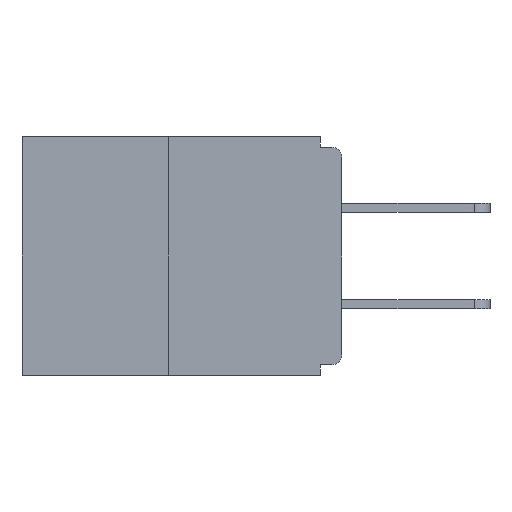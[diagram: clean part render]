
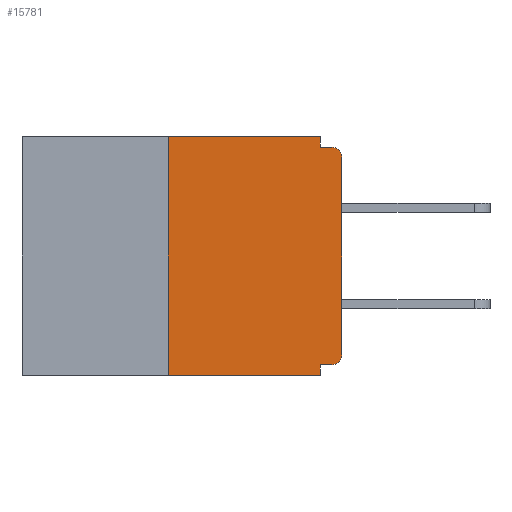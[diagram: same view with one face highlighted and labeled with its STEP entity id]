
A CAD part, left-side view. The second image highlights one B-rep face of the part: STEP entity #15781.
In plain terms, the highlighted planar face has unit normal (-1, 0, 0).
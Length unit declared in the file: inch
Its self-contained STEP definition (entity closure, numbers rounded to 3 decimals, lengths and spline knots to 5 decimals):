
#183 = CARTESIAN_POINT ( 'NONE',  ( 0., 0.46, 0. ) ) ;
#413 = ORIENTED_EDGE ( 'NONE', *, *, #6969, .F. ) ;
#437 = DIRECTION ( 'NONE',  ( 0., 0., -1. ) ) ;
#594 = VECTOR ( 'NONE', #13583, 39.37008 ) ;
#1017 = CIRCLE ( 'NONE', #13633, 0.015 ) ;
#1108 = VERTEX_POINT ( 'NONE', #19382 ) ;
#1325 = CARTESIAN_POINT ( 'NONE',  ( 0., 0.46, 0. ) ) ;
#1712 = FACE_OUTER_BOUND ( 'NONE', #11593, .T. ) ;
#1783 = PLANE ( 'NONE',  #17077 ) ;
#1824 = CARTESIAN_POINT ( 'NONE',  ( 0., 0., -0.015 ) ) ;
#2771 = CARTESIAN_POINT ( 'NONE',  ( 0., 0., 0. ) ) ;
#2826 = CARTESIAN_POINT ( 'NONE',  ( 0., 0.015, -0.03 ) ) ;
#3890 = ORIENTED_EDGE ( 'NONE', *, *, #14543, .F. ) ;
#4181 = EDGE_CURVE ( 'NONE', #9785, #1108, #5140, .T. ) ;
#4835 = CARTESIAN_POINT ( 'NONE',  ( 0., 0.031, 0. ) ) ;
#5004 = CARTESIAN_POINT ( 'NONE',  ( 0., 0.031, -0.328 ) ) ;
#5140 = LINE ( 'NONE', #2771, #10177 ) ;
#5144 = LINE ( 'NONE', #1824, #17123 ) ;
#6903 = VECTOR ( 'NONE', #10868, 39.37008 ) ;
#6969 = EDGE_CURVE ( 'NONE', #14451, #9485, #12203, .T. ) ;
#7129 = VERTEX_POINT ( 'NONE', #18935 ) ;
#7306 = VECTOR ( 'NONE', #13281, 39.37008 ) ;
#7949 = DIRECTION ( 'NONE',  ( 0., 0., -1. ) ) ;
#7967 = ORIENTED_EDGE ( 'NONE', *, *, #14686, .F. ) ;
#8321 = VERTEX_POINT ( 'NONE', #12087 ) ;
#8353 = CARTESIAN_POINT ( 'NONE',  ( 0., 0.031, 0. ) ) ;
#8525 = EDGE_CURVE ( 'NONE', #9485, #16801, #18585, .T. ) ;
#8793 = CARTESIAN_POINT ( 'NONE',  ( 0., 0., -0.313 ) ) ;
#9000 = EDGE_CURVE ( 'NONE', #19195, #7129, #12883, .T. ) ;
#9148 = ORIENTED_EDGE ( 'NONE', *, *, #10459, .T. ) ;
#9485 = VERTEX_POINT ( 'NONE', #4835 ) ;
#9785 = VERTEX_POINT ( 'NONE', #8793 ) ;
#10020 = LINE ( 'NONE', #18550, #6903 ) ;
#10177 = VECTOR ( 'NONE', #16263, 39.37008 ) ;
#10369 = ORIENTED_EDGE ( 'NONE', *, *, #8525, .F. ) ;
#10459 = EDGE_CURVE ( 'NONE', #1108, #12998, #18744, .T. ) ;
#10498 = ORIENTED_EDGE ( 'NONE', *, *, #13347, .F. ) ;
#10610 = CARTESIAN_POINT ( 'NONE',  ( 0., 0.25, 0. ) ) ;
#10640 = ORIENTED_EDGE ( 'NONE', *, *, #15071, .T. ) ;
#10708 = VECTOR ( 'NONE', #16726, 39.37008 ) ;
#10868 = DIRECTION ( 'NONE',  ( 0., -1., 0. ) ) ;
#11593 = EDGE_LOOP ( 'NONE', ( #413, #3890, #13366, #19313, #10498, #10640, #19316, #9148, #7967, #10369 ) ) ;
#11612 = AXIS2_PLACEMENT_3D ( 'NONE', #2826, #19827, #12222 ) ;
#12020 = CARTESIAN_POINT ( 'NONE',  ( 0., 0.25, 0. ) ) ;
#12087 = CARTESIAN_POINT ( 'NONE',  ( 0., 0.25, -0.343 ) ) ;
#12203 = LINE ( 'NONE', #1325, #16530 ) ;
#12222 = DIRECTION ( 'NONE',  ( 0., 0., -1. ) ) ;
#12266 = CARTESIAN_POINT ( 'NONE',  ( 0., 0.031, -0.015 ) ) ;
#12389 = CARTESIAN_POINT ( 'NONE',  ( 0., 0.015, -0.328 ) ) ;
#12601 = DIRECTION ( 'NONE',  ( 1., 0., 0. ) ) ;
#12847 = LINE ( 'NONE', #12020, #594 ) ;
#12883 = LINE ( 'NONE', #14752, #7306 ) ;
#12998 = VERTEX_POINT ( 'NONE', #18273 ) ;
#13281 = DIRECTION ( 'NONE',  ( 0., 0., -1. ) ) ;
#13347 = EDGE_CURVE ( 'NONE', #17828, #19195, #14816, .T. ) ;
#13366 = ORIENTED_EDGE ( 'NONE', *, *, #18509, .T. ) ;
#13583 = DIRECTION ( 'NONE',  ( 0., 0., 1. ) ) ;
#13633 = AXIS2_PLACEMENT_3D ( 'NONE', #18276, #16622, #19668 ) ;
#14066 = DIRECTION ( 'NONE',  ( 0., -1., 0. ) ) ;
#14451 = VERTEX_POINT ( 'NONE', #10610 ) ;
#14543 = EDGE_CURVE ( 'NONE', #8321, #14451, #12847, .T. ) ;
#14686 = EDGE_CURVE ( 'NONE', #16801, #12998, #5144, .T. ) ;
#14752 = CARTESIAN_POINT ( 'NONE',  ( 0., 0.031, -0.343 ) ) ;
#14816 = LINE ( 'NONE', #14874, #10708 ) ;
#14874 = CARTESIAN_POINT ( 'NONE',  ( 0., 0., -0.328 ) ) ;
#15071 = EDGE_CURVE ( 'NONE', #17828, #9785, #1017, .T. ) ;
#15781 = ADVANCED_FACE ( 'NONE', ( #1712 ), #1783, .F. ) ;
#16224 = VECTOR ( 'NONE', #437, 39.37008 ) ;
#16263 = DIRECTION ( 'NONE',  ( 0., 0., 1. ) ) ;
#16530 = VECTOR ( 'NONE', #18211, 39.37008 ) ;
#16622 = DIRECTION ( 'NONE',  ( -1., 0., 0. ) ) ;
#16726 = DIRECTION ( 'NONE',  ( 0., 1., 0. ) ) ;
#16801 = VERTEX_POINT ( 'NONE', #12266 ) ;
#17077 = AXIS2_PLACEMENT_3D ( 'NONE', #183, #12601, #7949 ) ;
#17123 = VECTOR ( 'NONE', #14066, 39.37008 ) ;
#17828 = VERTEX_POINT ( 'NONE', #12389 ) ;
#18211 = DIRECTION ( 'NONE',  ( 0., -1., 0. ) ) ;
#18273 = CARTESIAN_POINT ( 'NONE',  ( 0., 0.015, -0.015 ) ) ;
#18276 = CARTESIAN_POINT ( 'NONE',  ( 0., 0.015, -0.313 ) ) ;
#18509 = EDGE_CURVE ( 'NONE', #8321, #7129, #10020, .T. ) ;
#18550 = CARTESIAN_POINT ( 'NONE',  ( 0., 0.46, -0.343 ) ) ;
#18585 = LINE ( 'NONE', #8353, #16224 ) ;
#18744 = CIRCLE ( 'NONE', #11612, 0.015 ) ;
#18935 = CARTESIAN_POINT ( 'NONE',  ( 0., 0.031, -0.343 ) ) ;
#19195 = VERTEX_POINT ( 'NONE', #5004 ) ;
#19313 = ORIENTED_EDGE ( 'NONE', *, *, #9000, .F. ) ;
#19316 = ORIENTED_EDGE ( 'NONE', *, *, #4181, .T. ) ;
#19382 = CARTESIAN_POINT ( 'NONE',  ( 0., 0., -0.03 ) ) ;
#19668 = DIRECTION ( 'NONE',  ( 0., 0., -1. ) ) ;
#19827 = DIRECTION ( 'NONE',  ( -1., 0., 0. ) ) ;
